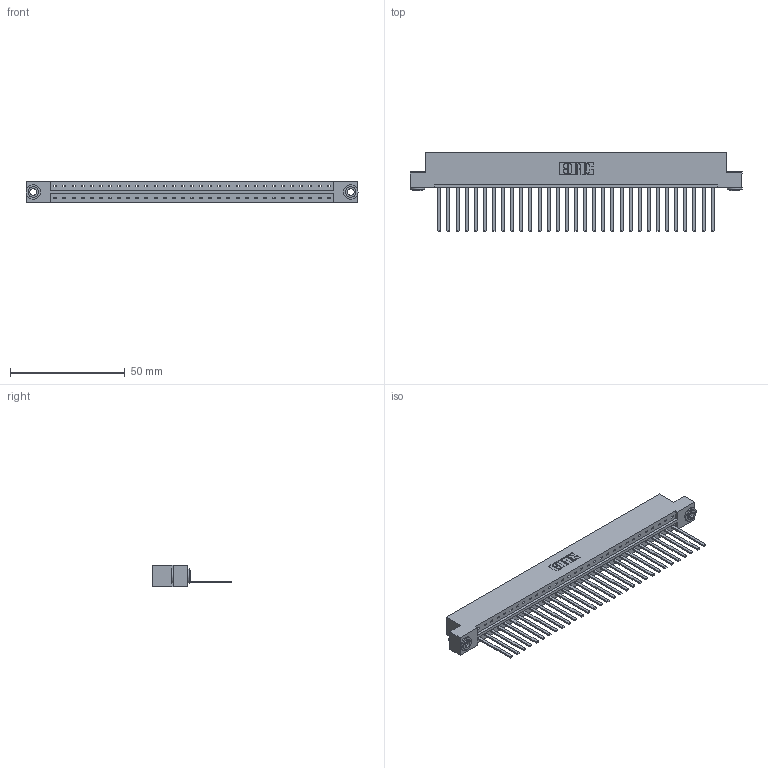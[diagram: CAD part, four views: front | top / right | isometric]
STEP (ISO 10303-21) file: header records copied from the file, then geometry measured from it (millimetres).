
FILE_DESCRIPTION (( 'STEP AP203' ), '1' );
FILE_NAME ('333-031-544-103.STEP', '2018-08-02T19:28:07', ( '' ), ( '' ), 'SwSTEP 2.0', 'SolidWorks 2016', '' );
FILE_SCHEMA (( 'CONFIG_CONTROL_DESIGN' ));
Length unit declared in the file: inch
Products named in the file (4): 345-250-002_345-250-002-102; 333-031-544-103; 333 Part_Flush - .156 Dia - TH; 345-292-001_345-293-144
Assembly tree (34 placements, depth 2):
  333-031-544-103
    333 Part_Flush - .156 Dia - TH
    345-292-001_345-293-144  x31
    345-250-002_345-250-002-102  x2
Bounding box: 144.37 x 34.3 x 9.4 mm (x, y, z)
Volume: 14811.9 mm3; surface area: 17349.2 mm2
Topology: 34 solids, 34 shells, 1764 faces, 5285 edges, 3478 vertices
Faces by surface type: plane 1258, cylinder 498, cone 8
Entity records: 20840 total; most frequent: CARTESIAN_POINT 3574, ORIENTED_EDGE 3534, DIRECTION 3067, EDGE_CURVE 1767, VECTOR 1619, LINE 1619, VERTEX_POINT 1174, AXIS2_PLACEMENT_3D 724
